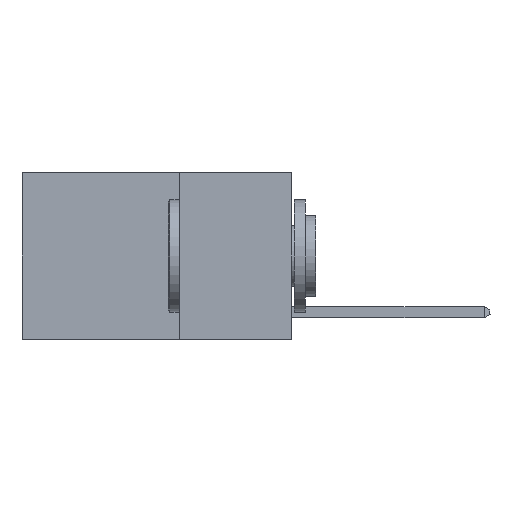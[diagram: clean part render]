
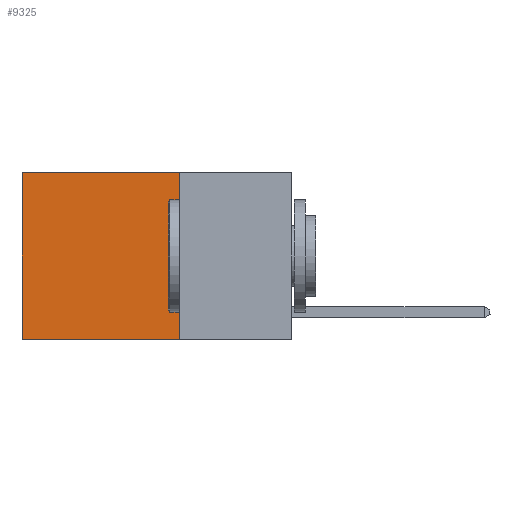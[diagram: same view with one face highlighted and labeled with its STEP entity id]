
A CAD part, left-side view. The second image highlights one B-rep face of the part: STEP entity #9325.
In plain terms, the highlighted planar face has unit normal (-1, 0, 0).
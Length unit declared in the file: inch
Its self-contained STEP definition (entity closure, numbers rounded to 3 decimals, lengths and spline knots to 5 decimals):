
#269 = LINE ( 'NONE', #5105, #3129 ) ;
#1623 = DIRECTION ( 'NONE',  ( 0., 0., -1. ) ) ;
#1655 = ORIENTED_EDGE ( 'NONE', *, *, #12083, .T. ) ;
#2158 = EDGE_LOOP ( 'NONE', ( #6579, #7218, #11040, #1655 ) ) ;
#2195 = DIRECTION ( 'NONE',  ( 0., 1., 0. ) ) ;
#3031 = CARTESIAN_POINT ( 'NONE',  ( 0.2625, 0.25, 0. ) ) ;
#3129 = VECTOR ( 'NONE', #6955, 39.37008 ) ;
#3246 = CARTESIAN_POINT ( 'NONE',  ( 0.2625, 0.25, -0.37 ) ) ;
#3727 = AXIS2_PLACEMENT_3D ( 'NONE', #11978, #9308, #9367 ) ;
#3735 = CARTESIAN_POINT ( 'NONE',  ( 0.2625, 0.25, -0.37 ) ) ;
#3928 = EDGE_CURVE ( 'NONE', #7213, #9721, #11570, .T. ) ;
#5070 = DIRECTION ( 'NONE',  ( 0., 1., 0. ) ) ;
#5105 = CARTESIAN_POINT ( 'NONE',  ( 0.2625, 0.25, 0. ) ) ;
#5538 = CARTESIAN_POINT ( 'NONE',  ( 0.2625, 0.6, -0.37 ) ) ;
#6235 = CARTESIAN_POINT ( 'NONE',  ( 0.2625, 0.6, 0. ) ) ;
#6579 = ORIENTED_EDGE ( 'NONE', *, *, #9819, .T. ) ;
#6634 = LINE ( 'NONE', #7451, #11575 ) ;
#6955 = DIRECTION ( 'NONE',  ( 0., 0., -1. ) ) ;
#7213 = VERTEX_POINT ( 'NONE', #3735 ) ;
#7218 = ORIENTED_EDGE ( 'NONE', *, *, #3928, .F. ) ;
#7408 = LINE ( 'NONE', #6235, #9979 ) ;
#7451 = CARTESIAN_POINT ( 'NONE',  ( 0.2625, 0.25, 0. ) ) ;
#7788 = VERTEX_POINT ( 'NONE', #3031 ) ;
#7883 = EDGE_CURVE ( 'NONE', #7788, #7213, #269, .T. ) ;
#8373 = VECTOR ( 'NONE', #2195, 39.37008 ) ;
#8876 = CARTESIAN_POINT ( 'NONE',  ( 0.2625, 0.6, 0. ) ) ;
#9178 = FACE_OUTER_BOUND ( 'NONE', #2158, .T. ) ;
#9308 = DIRECTION ( 'NONE',  ( 1., 0., 0. ) ) ;
#9325 = ADVANCED_FACE ( 'NONE', ( #9178 ), #11123, .F. ) ;
#9367 = DIRECTION ( 'NONE',  ( 0., 0., -1. ) ) ;
#9721 = VERTEX_POINT ( 'NONE', #5538 ) ;
#9819 = EDGE_CURVE ( 'NONE', #12098, #9721, #7408, .T. ) ;
#9979 = VECTOR ( 'NONE', #1623, 39.37008 ) ;
#11040 = ORIENTED_EDGE ( 'NONE', *, *, #7883, .F. ) ;
#11123 = PLANE ( 'NONE',  #3727 ) ;
#11570 = LINE ( 'NONE', #3246, #8373 ) ;
#11575 = VECTOR ( 'NONE', #5070, 39.37008 ) ;
#11978 = CARTESIAN_POINT ( 'NONE',  ( 0.2625, 0.25, 0. ) ) ;
#12083 = EDGE_CURVE ( 'NONE', #7788, #12098, #6634, .T. ) ;
#12098 = VERTEX_POINT ( 'NONE', #8876 ) ;
